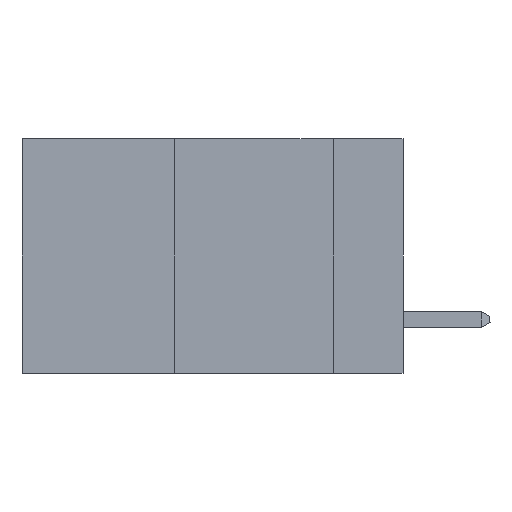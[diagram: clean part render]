
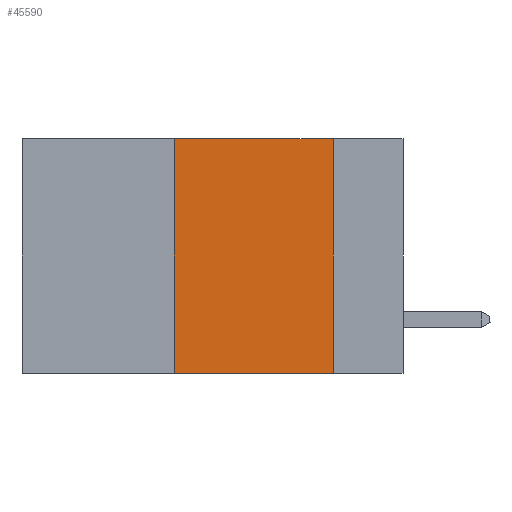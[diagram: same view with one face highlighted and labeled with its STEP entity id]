
A CAD part, left-side view. The second image highlights one B-rep face of the part: STEP entity #45590.
In plain terms, the highlighted planar face has unit normal (-1, 0, 0).
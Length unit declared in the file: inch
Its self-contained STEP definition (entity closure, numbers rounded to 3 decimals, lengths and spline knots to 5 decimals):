
#415 = VERTEX_POINT ( 'NONE', #7620 ) ;
#1367 = CARTESIAN_POINT ( 'NONE',  ( 0., 0.6, 0. ) ) ;
#1844 = DIRECTION ( 'NONE',  ( 1., 0., 0. ) ) ;
#1921 = ORIENTED_EDGE ( 'NONE', *, *, #46579, .F. ) ;
#3478 = CARTESIAN_POINT ( 'NONE',  ( 0., 0.6, -0.37 ) ) ;
#4604 = FACE_OUTER_BOUND ( 'NONE', #30188, .T. ) ;
#7620 = CARTESIAN_POINT ( 'NONE',  ( 0., 0.36, -0.37 ) ) ;
#9444 = VERTEX_POINT ( 'NONE', #46339 ) ;
#14942 = LINE ( 'NONE', #41224, #19666 ) ;
#15787 = CARTESIAN_POINT ( 'NONE',  ( 0., 0.6, 0. ) ) ;
#15904 = ORIENTED_EDGE ( 'NONE', *, *, #39414, .F. ) ;
#16105 = CARTESIAN_POINT ( 'NONE',  ( 0., 0.36, 0. ) ) ;
#18063 = DIRECTION ( 'NONE',  ( 0., 0., -1. ) ) ;
#19666 = VECTOR ( 'NONE', #18063, 39.37008 ) ;
#20189 = PLANE ( 'NONE',  #39431 ) ;
#21729 = EDGE_CURVE ( 'NONE', #24079, #9444, #14942, .T. ) ;
#23534 = EDGE_CURVE ( 'NONE', #415, #9444, #25398, .T. ) ;
#24079 = VERTEX_POINT ( 'NONE', #40841 ) ;
#24660 = VERTEX_POINT ( 'NONE', #29082 ) ;
#25398 = LINE ( 'NONE', #3478, #26577 ) ;
#26577 = VECTOR ( 'NONE', #36776, 39.37008 ) ;
#28043 = DIRECTION ( 'NONE',  ( 0., 0., -1. ) ) ;
#29082 = CARTESIAN_POINT ( 'NONE',  ( 0., 0.36, 0. ) ) ;
#29760 = VECTOR ( 'NONE', #30667, 39.37008 ) ;
#30188 = EDGE_LOOP ( 'NONE', ( #43240, #1921, #15904, #35790 ) ) ;
#30667 = DIRECTION ( 'NONE',  ( 0., -1., 0. ) ) ;
#32079 = LINE ( 'NONE', #16105, #36826 ) ;
#35790 = ORIENTED_EDGE ( 'NONE', *, *, #23534, .T. ) ;
#36776 = DIRECTION ( 'NONE',  ( 0., -1., 0. ) ) ;
#36826 = VECTOR ( 'NONE', #38756, 39.37008 ) ;
#38756 = DIRECTION ( 'NONE',  ( 0., 0., 1. ) ) ;
#39414 = EDGE_CURVE ( 'NONE', #415, #24660, #32079, .T. ) ;
#39431 = AXIS2_PLACEMENT_3D ( 'NONE', #1367, #1844, #28043 ) ;
#40841 = CARTESIAN_POINT ( 'NONE',  ( 0., 0.11, 0. ) ) ;
#41224 = CARTESIAN_POINT ( 'NONE',  ( 0., 0.11, 0. ) ) ;
#43240 = ORIENTED_EDGE ( 'NONE', *, *, #21729, .F. ) ;
#45590 = ADVANCED_FACE ( 'NONE', ( #4604 ), #20189, .F. ) ;
#46339 = CARTESIAN_POINT ( 'NONE',  ( 0., 0.11, -0.37 ) ) ;
#46579 = EDGE_CURVE ( 'NONE', #24660, #24079, #47374, .T. ) ;
#47374 = LINE ( 'NONE', #15787, #29760 ) ;
